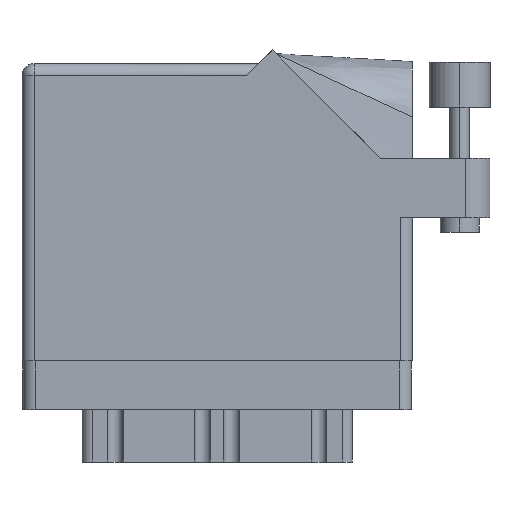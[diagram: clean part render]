
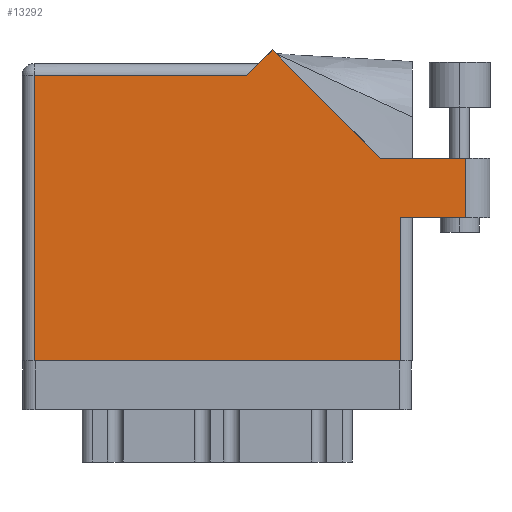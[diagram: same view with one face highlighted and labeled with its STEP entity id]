
A CAD part, front view. The second image highlights one B-rep face of the part: STEP entity #13292.
In plain terms, the highlighted face is planar.
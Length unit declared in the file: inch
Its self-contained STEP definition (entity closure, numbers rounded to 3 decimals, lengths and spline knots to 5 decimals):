
#133 = LINE ( 'NONE', #34509, #16982 ) ;
#157 = EDGE_CURVE ( 'NONE', #2098, #1173, #17283, .T. ) ;
#519 = CARTESIAN_POINT ( 'NONE',  ( 1.84442, 1.044, 0. ) ) ;
#536 = VERTEX_POINT ( 'NONE', #1307 ) ;
#972 = DIRECTION ( 'NONE',  ( -1., 0., 0. ) ) ;
#1173 = VERTEX_POINT ( 'NONE', #12480 ) ;
#1307 = CARTESIAN_POINT ( 'NONE',  ( 1.155, 1.468, 0. ) ) ;
#1371 = EDGE_CURVE ( 'NONE', #20713, #9743, #6140, .T. ) ;
#2098 = VERTEX_POINT ( 'NONE', #23773 ) ;
#2176 = ORIENTED_EDGE ( 'NONE', *, *, #1371, .T. ) ;
#2856 = LINE ( 'NONE', #27214, #33562 ) ;
#3087 = CARTESIAN_POINT ( 'NONE',  ( 1.84442, 1.044, 0. ) ) ;
#3264 = VECTOR ( 'NONE', #30970, 39.37008 ) ;
#3854 = PLANE ( 'NONE',  #33647 ) ;
#4740 = DIRECTION ( 'NONE',  ( -0.707, -0.707, 0. ) ) ;
#5059 = VERTEX_POINT ( 'NONE', #25920 ) ;
#6140 = LINE ( 'NONE', #519, #30289 ) ;
#6666 = CARTESIAN_POINT ( 'NONE',  ( 0., 1.53, 0. ) ) ;
#7303 = ORIENTED_EDGE ( 'NONE', *, *, #157, .T. ) ;
#7541 = VECTOR ( 'NONE', #4740, 39.37008 ) ;
#7665 = VECTOR ( 'NONE', #28134, 39.37008 ) ;
#7773 = DIRECTION ( 'NONE',  ( -1., 0., 0. ) ) ;
#8039 = EDGE_CURVE ( 'NONE', #19772, #5059, #133, .T. ) ;
#8334 = LINE ( 'NONE', #29532, #24936 ) ;
#8407 = VERTEX_POINT ( 'NONE', #10322 ) ;
#9146 = ORIENTED_EDGE ( 'NONE', *, *, #19424, .T. ) ;
#9743 = VERTEX_POINT ( 'NONE', #28894 ) ;
#10322 = CARTESIAN_POINT ( 'NONE',  ( 0.062, 1.468, 0. ) ) ;
#10408 = EDGE_CURVE ( 'NONE', #5059, #18330, #14661, .T. ) ;
#11104 = DIRECTION ( 'NONE',  ( 0., -1., 0. ) ) ;
#11227 = DIRECTION ( 'NONE',  ( -0.707, 0.707, 0. ) ) ;
#12164 = EDGE_LOOP ( 'NONE', ( #23113, #7303, #32308, #2176, #18426, #9146, #34648, #26489, #33506 ) ) ;
#12480 = CARTESIAN_POINT ( 'NONE',  ( 2.285, 1.044, 0. ) ) ;
#12646 = CARTESIAN_POINT ( 'NONE',  ( 1.217, 1.53, 0. ) ) ;
#13292 = ADVANCED_FACE ( 'NONE', ( #33459 ), #3854, .F. ) ;
#14661 = LINE ( 'NONE', #17456, #7665 ) ;
#15499 = LINE ( 'NONE', #31260, #23360 ) ;
#15803 = EDGE_CURVE ( 'NONE', #8407, #19772, #2856, .T. ) ;
#16982 = VECTOR ( 'NONE', #29067, 39.37008 ) ;
#17283 = LINE ( 'NONE', #22702, #24623 ) ;
#17456 = CARTESIAN_POINT ( 'NONE',  ( 1.948, 0.737, 0. ) ) ;
#18247 = LINE ( 'NONE', #12646, #7541 ) ;
#18294 = CARTESIAN_POINT ( 'NONE',  ( 0.062, 0., 0. ) ) ;
#18330 = VERTEX_POINT ( 'NONE', #30394 ) ;
#18426 = ORIENTED_EDGE ( 'NONE', *, *, #18883, .T. ) ;
#18883 = EDGE_CURVE ( 'NONE', #9743, #536, #18247, .T. ) ;
#19424 = EDGE_CURVE ( 'NONE', #536, #8407, #8334, .T. ) ;
#19643 = DIRECTION ( 'NONE',  ( -1., 0., 0. ) ) ;
#19772 = VERTEX_POINT ( 'NONE', #18294 ) ;
#20116 = LINE ( 'NONE', #20281, #3264 ) ;
#20281 = CARTESIAN_POINT ( 'NONE',  ( 2.01, 0.737, 0. ) ) ;
#20713 = VERTEX_POINT ( 'NONE', #3087 ) ;
#22647 = EDGE_CURVE ( 'NONE', #1173, #20713, #15499, .T. ) ;
#22702 = CARTESIAN_POINT ( 'NONE',  ( 2.285, 1.044, 0. ) ) ;
#23113 = ORIENTED_EDGE ( 'NONE', *, *, #23914, .T. ) ;
#23360 = VECTOR ( 'NONE', #7773, 39.37008 ) ;
#23773 = CARTESIAN_POINT ( 'NONE',  ( 2.285, 0.737, 0. ) ) ;
#23914 = EDGE_CURVE ( 'NONE', #18330, #2098, #20116, .T. ) ;
#24623 = VECTOR ( 'NONE', #27959, 39.37008 ) ;
#24936 = VECTOR ( 'NONE', #972, 39.37008 ) ;
#25920 = CARTESIAN_POINT ( 'NONE',  ( 1.948, 0., 0. ) ) ;
#26489 = ORIENTED_EDGE ( 'NONE', *, *, #8039, .T. ) ;
#27214 = CARTESIAN_POINT ( 'NONE',  ( 0.062, 0., 0. ) ) ;
#27959 = DIRECTION ( 'NONE',  ( 0., 1., 0. ) ) ;
#28039 = DIRECTION ( 'NONE',  ( 0., 0., -1. ) ) ;
#28134 = DIRECTION ( 'NONE',  ( 0., 1., 0. ) ) ;
#28894 = CARTESIAN_POINT ( 'NONE',  ( 1.28771, 1.60071, 0. ) ) ;
#29067 = DIRECTION ( 'NONE',  ( 1., 0., 0. ) ) ;
#29532 = CARTESIAN_POINT ( 'NONE',  ( 0., 1.468, 0. ) ) ;
#30289 = VECTOR ( 'NONE', #11227, 39.37008 ) ;
#30394 = CARTESIAN_POINT ( 'NONE',  ( 1.948, 0.737, 0. ) ) ;
#30970 = DIRECTION ( 'NONE',  ( 1., 0., 0. ) ) ;
#31260 = CARTESIAN_POINT ( 'NONE',  ( 2.41, 1.044, 0. ) ) ;
#32308 = ORIENTED_EDGE ( 'NONE', *, *, #22647, .T. ) ;
#33459 = FACE_OUTER_BOUND ( 'NONE', #12164, .T. ) ;
#33506 = ORIENTED_EDGE ( 'NONE', *, *, #10408, .T. ) ;
#33562 = VECTOR ( 'NONE', #11104, 39.37008 ) ;
#33647 = AXIS2_PLACEMENT_3D ( 'NONE', #6666, #28039, #19643 ) ;
#34509 = CARTESIAN_POINT ( 'NONE',  ( 0., 0., 0. ) ) ;
#34648 = ORIENTED_EDGE ( 'NONE', *, *, #15803, .T. ) ;
